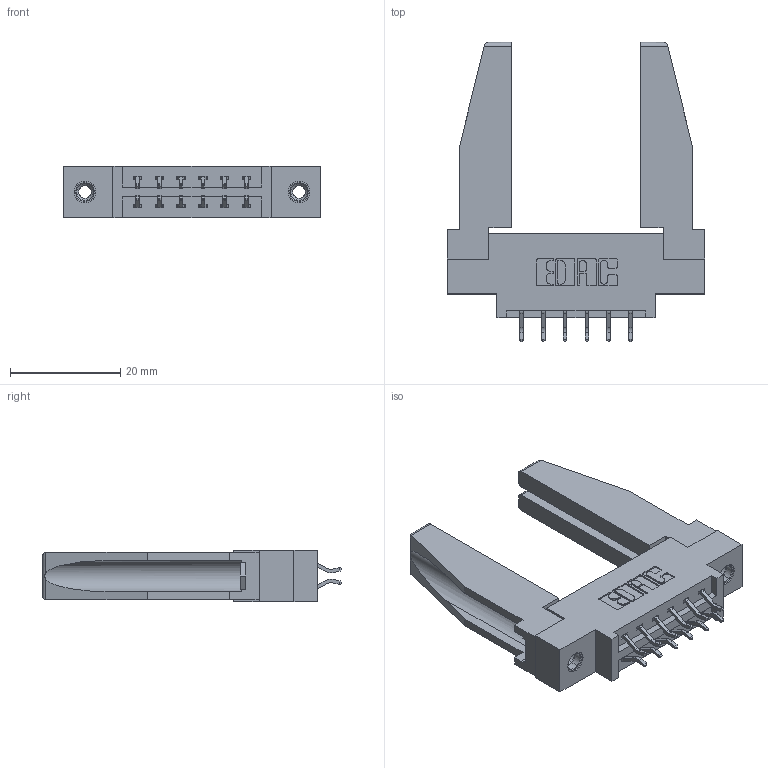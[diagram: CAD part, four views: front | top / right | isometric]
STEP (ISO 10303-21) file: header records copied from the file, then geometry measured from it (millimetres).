
FILE_DESCRIPTION (( 'STEP AP203' ), '1' );
FILE_NAME ('337-012-556-878.STEP', '2019-10-10T16:21:13', ( '' ), ( '' ), 'SwSTEP 2.0', 'SolidWorks 2016', '' );
FILE_SCHEMA (( 'CONFIG_CONTROL_DESIGN' ));
Length unit declared in the file: inch
Products named in the file (5): 337-012-556-878; 345-250-001_345-250-001-102; 345-292-001_556 Tail; 337 Part_0.170 Offset - 0.156 Dia-TI; 307-220-078
Assembly tree (17 placements, depth 2):
  337-012-556-878
    337 Part_0.170 Offset - 0.156 Dia-TI
    345-292-001_556 Tail  x12
    345-250-001_345-250-001-102  x2
    307-220-078  x2
Bounding box: 46.79 x 54.37 x 9.4 mm (x, y, z)
Volume: 8326.9 mm3; surface area: 8475.1 mm2
Topology: 17 solids, 17 shells, 968 faces, 2801 edges, 1842 vertices
Faces by surface type: plane 662, cylinder 290, cone 12, torus 4
Entity records: 12100 total; most frequent: CARTESIAN_POINT 2084, ORIENTED_EDGE 1964, DIRECTION 1834, EDGE_CURVE 982, VECTOR 808, LINE 808, VERTEX_POINT 648, AXIS2_PLACEMENT_3D 513
